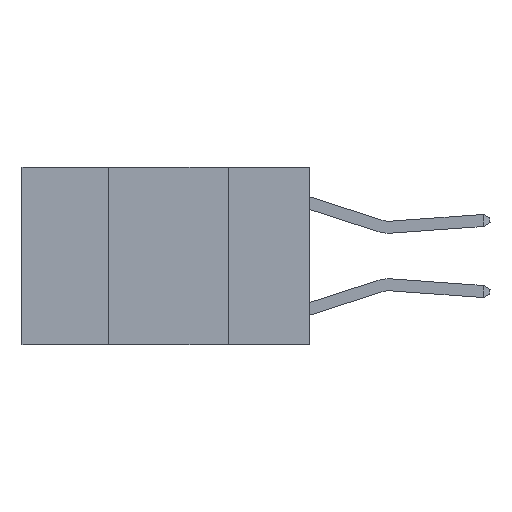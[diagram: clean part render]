
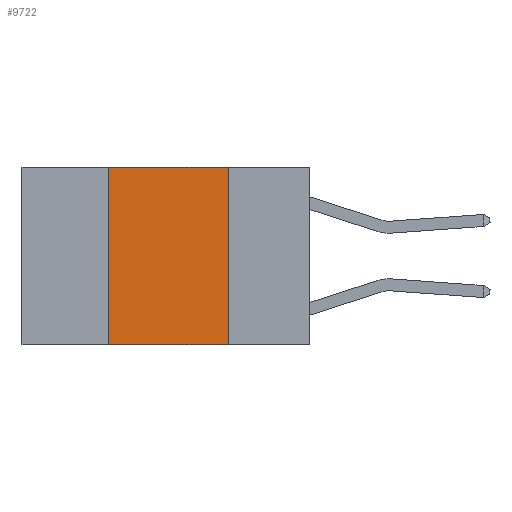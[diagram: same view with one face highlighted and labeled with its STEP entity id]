
A CAD part, left-side view. The second image highlights one B-rep face of the part: STEP entity #9722.
In plain terms, the highlighted planar face has unit normal (-1, 0, 0).
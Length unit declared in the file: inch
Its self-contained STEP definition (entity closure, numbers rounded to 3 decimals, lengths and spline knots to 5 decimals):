
#695 = LINE ( 'NONE', #8206, #12828 ) ;
#853 = VERTEX_POINT ( 'NONE', #3089 ) ;
#886 = ORIENTED_EDGE ( 'NONE', *, *, #7325, .F. ) ;
#1373 = CARTESIAN_POINT ( 'NONE',  ( 0., 0.42, -0.37 ) ) ;
#1532 = CARTESIAN_POINT ( 'NONE',  ( 0., 0.17, 0. ) ) ;
#1654 = EDGE_CURVE ( 'NONE', #9837, #11688, #695, .T. ) ;
#1866 = DIRECTION ( 'NONE',  ( 0., 0., -1. ) ) ;
#2106 = VECTOR ( 'NONE', #9757, 39.37008 ) ;
#3089 = CARTESIAN_POINT ( 'NONE',  ( 0., 0.42, 0. ) ) ;
#3565 = DIRECTION ( 'NONE',  ( 0., 0., -1. ) ) ;
#3897 = DIRECTION ( 'NONE',  ( 0., 0., 1. ) ) ;
#4012 = DIRECTION ( 'NONE',  ( 0., -1., 0. ) ) ;
#5100 = CARTESIAN_POINT ( 'NONE',  ( 0., 0.42, 0. ) ) ;
#5147 = EDGE_CURVE ( 'NONE', #6869, #11688, #9051, .T. ) ;
#5167 = ORIENTED_EDGE ( 'NONE', *, *, #1654, .T. ) ;
#6869 = VERTEX_POINT ( 'NONE', #1532 ) ;
#7023 = CARTESIAN_POINT ( 'NONE',  ( 0., 0.17, -0.37 ) ) ;
#7197 = AXIS2_PLACEMENT_3D ( 'NONE', #9022, #8816, #3565 ) ;
#7325 = EDGE_CURVE ( 'NONE', #9837, #853, #10597, .T. ) ;
#7835 = ORIENTED_EDGE ( 'NONE', *, *, #10178, .F. ) ;
#8021 = EDGE_LOOP ( 'NONE', ( #13557, #7835, #886, #5167 ) ) ;
#8206 = CARTESIAN_POINT ( 'NONE',  ( 0., 0.6, -0.37 ) ) ;
#8816 = DIRECTION ( 'NONE',  ( 1., 0., 0. ) ) ;
#9022 = CARTESIAN_POINT ( 'NONE',  ( 0., 0.6, 0. ) ) ;
#9051 = LINE ( 'NONE', #9125, #12615 ) ;
#9125 = CARTESIAN_POINT ( 'NONE',  ( 0., 0.17, 0. ) ) ;
#9618 = LINE ( 'NONE', #11913, #2106 ) ;
#9722 = ADVANCED_FACE ( 'NONE', ( #12298 ), #13327, .F. ) ;
#9757 = DIRECTION ( 'NONE',  ( 0., -1., 0. ) ) ;
#9837 = VERTEX_POINT ( 'NONE', #1373 ) ;
#10178 = EDGE_CURVE ( 'NONE', #853, #6869, #9618, .T. ) ;
#10597 = LINE ( 'NONE', #5100, #13123 ) ;
#11688 = VERTEX_POINT ( 'NONE', #7023 ) ;
#11913 = CARTESIAN_POINT ( 'NONE',  ( 0., 0.6, 0. ) ) ;
#12298 = FACE_OUTER_BOUND ( 'NONE', #8021, .T. ) ;
#12615 = VECTOR ( 'NONE', #1866, 39.37008 ) ;
#12828 = VECTOR ( 'NONE', #4012, 39.37008 ) ;
#13123 = VECTOR ( 'NONE', #3897, 39.37008 ) ;
#13327 = PLANE ( 'NONE',  #7197 ) ;
#13557 = ORIENTED_EDGE ( 'NONE', *, *, #5147, .F. ) ;
